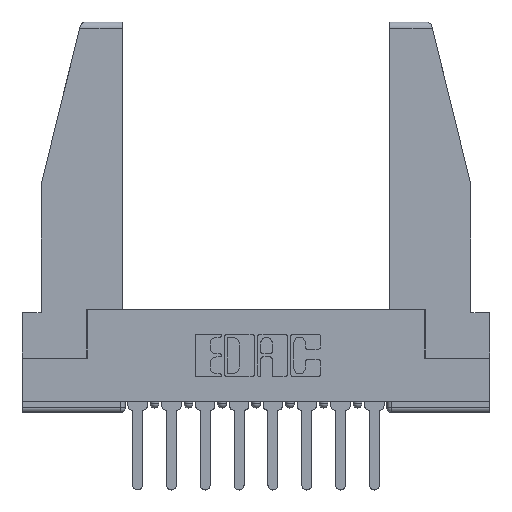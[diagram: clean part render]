
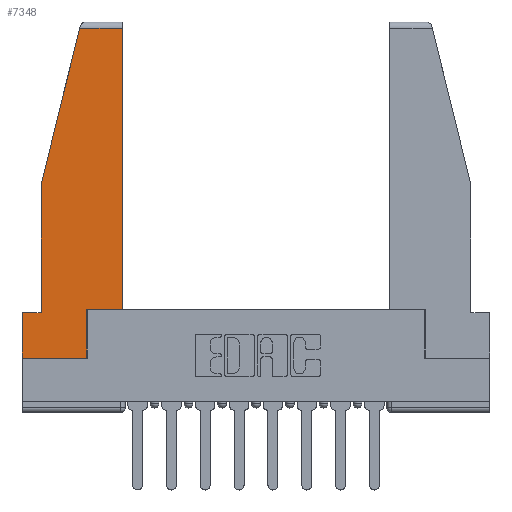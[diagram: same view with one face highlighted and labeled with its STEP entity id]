
A CAD part, top view. The second image highlights one B-rep face of the part: STEP entity #7348.
In plain terms, the highlighted planar face has unit normal (0, 0, 1).
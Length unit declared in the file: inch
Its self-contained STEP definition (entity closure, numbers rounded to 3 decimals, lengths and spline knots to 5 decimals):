
#38 = DIRECTION ( 'NONE',  ( 1., 0., 0. ) ) ;
#216 = VERTEX_POINT ( 'NONE', #6684 ) ;
#907 = LINE ( 'NONE', #9265, #12876 ) ;
#917 = CARTESIAN_POINT ( 'NONE',  ( 0., 0., 0. ) ) ;
#979 = VERTEX_POINT ( 'NONE', #11305 ) ;
#1054 = LINE ( 'NONE', #5316, #7476 ) ;
#1465 = CARTESIAN_POINT ( 'NONE',  ( 0.086, 0.8, 0. ) ) ;
#1704 = VERTEX_POINT ( 'NONE', #1465 ) ;
#1831 = ORIENTED_EDGE ( 'NONE', *, *, #10213, .T. ) ;
#1849 = VECTOR ( 'NONE', #38, 39.37008 ) ;
#1991 = FACE_OUTER_BOUND ( 'NONE', #3402, .T. ) ;
#2131 = ORIENTED_EDGE ( 'NONE', *, *, #7080, .T. ) ;
#2444 = CARTESIAN_POINT ( 'NONE',  ( 0.086, 0.8, 0. ) ) ;
#2558 = CARTESIAN_POINT ( 'NONE',  ( 0.461, 0.223, 0. ) ) ;
#2735 = LINE ( 'NONE', #2444, #6963 ) ;
#2920 = ORIENTED_EDGE ( 'NONE', *, *, #5473, .T. ) ;
#3096 = CARTESIAN_POINT ( 'NONE',  ( 0.461, 0.223, 0. ) ) ;
#3114 = VERTEX_POINT ( 'NONE', #11756 ) ;
#3317 = LINE ( 'NONE', #7567, #1849 ) ;
#3402 = EDGE_LOOP ( 'NONE', ( #1831, #12283, #2131, #5354, #7344, #2920, #4399, #8645, #9099 ) ) ;
#3978 = EDGE_CURVE ( 'NONE', #3999, #979, #8947, .T. ) ;
#3999 = VERTEX_POINT ( 'NONE', #4442 ) ;
#4284 = AXIS2_PLACEMENT_3D ( 'NONE', #6246, #6043, #10291 ) ;
#4399 = ORIENTED_EDGE ( 'NONE', *, *, #8745, .T. ) ;
#4442 = CARTESIAN_POINT ( 'NONE',  ( 0.086, 0.21, 0. ) ) ;
#4511 = CARTESIAN_POINT ( 'NONE',  ( 0.461, 1.52, 0. ) ) ;
#4535 = EDGE_CURVE ( 'NONE', #13106, #11465, #907, .T. ) ;
#5316 = CARTESIAN_POINT ( 'NONE',  ( 0.297, 0.223, 0. ) ) ;
#5354 = ORIENTED_EDGE ( 'NONE', *, *, #8073, .T. ) ;
#5371 = EDGE_CURVE ( 'NONE', #3114, #216, #7028, .T. ) ;
#5473 = EDGE_CURVE ( 'NONE', #979, #12174, #13398, .T. ) ;
#6043 = DIRECTION ( 'NONE',  ( 0., 0., 1. ) ) ;
#6119 = DIRECTION ( 'NONE',  ( 0., 1., 0. ) ) ;
#6153 = DIRECTION ( 'NONE',  ( -1., 0., 0. ) ) ;
#6246 = CARTESIAN_POINT ( 'NONE',  ( 0., 0., 0. ) ) ;
#6251 = DIRECTION ( 'NONE',  ( 0., -1., 0. ) ) ;
#6458 = CARTESIAN_POINT ( 'NONE',  ( 0., 0.21, 0. ) ) ;
#6684 = CARTESIAN_POINT ( 'NONE',  ( 0.297, 0.223, 0. ) ) ;
#6743 = VECTOR ( 'NONE', #10001, 39.37008 ) ;
#6963 = VECTOR ( 'NONE', #7792, 39.37008 ) ;
#7028 = LINE ( 'NONE', #9093, #9127 ) ;
#7080 = EDGE_CURVE ( 'NONE', #11465, #1704, #8868, .T. ) ;
#7092 = PLANE ( 'NONE',  #4284 ) ;
#7344 = ORIENTED_EDGE ( 'NONE', *, *, #3978, .T. ) ;
#7348 = ADVANCED_FACE ( 'NONE', ( #1991 ), #7092, .T. ) ;
#7476 = VECTOR ( 'NONE', #12732, 39.37008 ) ;
#7567 = CARTESIAN_POINT ( 'NONE',  ( 0., 0., 0. ) ) ;
#7706 = DIRECTION ( 'NONE',  ( -1., 0., 0. ) ) ;
#7792 = DIRECTION ( 'NONE',  ( 0., -1., 0. ) ) ;
#7986 = VECTOR ( 'NONE', #7706, 39.37008 ) ;
#8073 = EDGE_CURVE ( 'NONE', #1704, #3999, #2735, .T. ) ;
#8109 = CARTESIAN_POINT ( 'NONE',  ( 0.271, 1.55, 0. ) ) ;
#8645 = ORIENTED_EDGE ( 'NONE', *, *, #5371, .T. ) ;
#8745 = EDGE_CURVE ( 'NONE', #12174, #3114, #3317, .T. ) ;
#8868 = LINE ( 'NONE', #8109, #6743 ) ;
#8871 = DIRECTION ( 'NONE',  ( 0., 1., 0. ) ) ;
#8947 = LINE ( 'NONE', #9808, #7986 ) ;
#9093 = CARTESIAN_POINT ( 'NONE',  ( 0.297, 0., 0. ) ) ;
#9099 = ORIENTED_EDGE ( 'NONE', *, *, #12237, .T. ) ;
#9127 = VECTOR ( 'NONE', #6119, 39.37008 ) ;
#9265 = CARTESIAN_POINT ( 'NONE',  ( 0., 1.52, 0. ) ) ;
#9572 = VECTOR ( 'NONE', #6251, 39.37008 ) ;
#9808 = CARTESIAN_POINT ( 'NONE',  ( 0., 0.21, 0. ) ) ;
#9879 = VECTOR ( 'NONE', #8871, 39.37008 ) ;
#10001 = DIRECTION ( 'NONE',  ( -0.239, -0.971, 0. ) ) ;
#10213 = EDGE_CURVE ( 'NONE', #11760, #13106, #11925, .T. ) ;
#10291 = DIRECTION ( 'NONE',  ( 1., 0., 0. ) ) ;
#11305 = CARTESIAN_POINT ( 'NONE',  ( 0., 0.21, 0. ) ) ;
#11465 = VERTEX_POINT ( 'NONE', #12193 ) ;
#11756 = CARTESIAN_POINT ( 'NONE',  ( 0.297, 0., 0. ) ) ;
#11760 = VERTEX_POINT ( 'NONE', #3096 ) ;
#11925 = LINE ( 'NONE', #2558, #9879 ) ;
#12174 = VERTEX_POINT ( 'NONE', #917 ) ;
#12193 = CARTESIAN_POINT ( 'NONE',  ( 0.2636, 1.52, 0. ) ) ;
#12237 = EDGE_CURVE ( 'NONE', #216, #11760, #1054, .T. ) ;
#12283 = ORIENTED_EDGE ( 'NONE', *, *, #4535, .T. ) ;
#12732 = DIRECTION ( 'NONE',  ( 1., 0., 0. ) ) ;
#12876 = VECTOR ( 'NONE', #6153, 39.37008 ) ;
#13106 = VERTEX_POINT ( 'NONE', #4511 ) ;
#13398 = LINE ( 'NONE', #6458, #9572 ) ;
